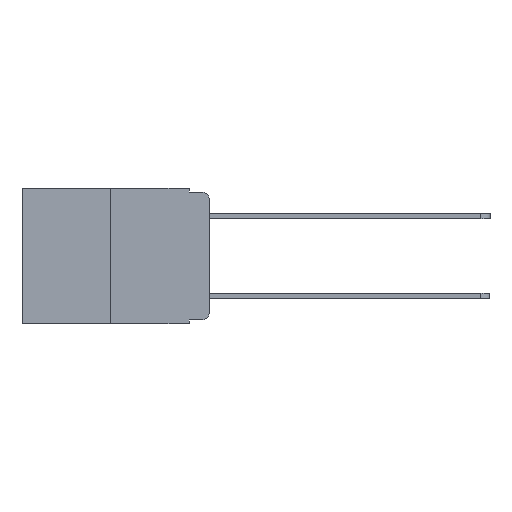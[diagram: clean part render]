
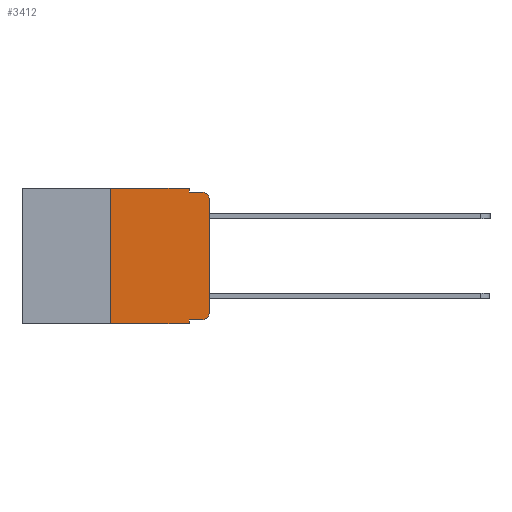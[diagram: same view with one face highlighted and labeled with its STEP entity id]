
A CAD part, left-side view. The second image highlights one B-rep face of the part: STEP entity #3412.
In plain terms, the highlighted planar face has unit normal (-1, 0, 0).
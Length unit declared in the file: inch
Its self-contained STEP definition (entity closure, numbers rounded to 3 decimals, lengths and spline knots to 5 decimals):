
#93 = LINE ( 'NONE', #2620, #12714 ) ;
#196 = CARTESIAN_POINT ( 'NONE',  ( 0., 0.051, -0.343 ) ) ;
#274 = VERTEX_POINT ( 'NONE', #10765 ) ;
#384 = LINE ( 'NONE', #11797, #10705 ) ;
#469 = CARTESIAN_POINT ( 'NONE',  ( 0., 0.051, -0.333 ) ) ;
#595 = VECTOR ( 'NONE', #872, 39.37008 ) ;
#602 = CARTESIAN_POINT ( 'NONE',  ( 0., 0.02, -0.03 ) ) ;
#603 = LINE ( 'NONE', #9924, #962 ) ;
#618 = EDGE_CURVE ( 'NONE', #274, #6680, #93, .T. ) ;
#852 = VERTEX_POINT ( 'NONE', #7088 ) ;
#872 = DIRECTION ( 'NONE',  ( 0., 0., -1. ) ) ;
#962 = VECTOR ( 'NONE', #9908, 39.37008 ) ;
#974 = CARTESIAN_POINT ( 'NONE',  ( 0., 0., -0.03 ) ) ;
#1253 = LINE ( 'NONE', #10570, #11458 ) ;
#1370 = EDGE_CURVE ( 'NONE', #6028, #9421, #603, .T. ) ;
#1397 = DIRECTION ( 'NONE',  ( 1., 0., 0. ) ) ;
#1731 = DIRECTION ( 'NONE',  ( 0., 0., -1. ) ) ;
#1858 = EDGE_CURVE ( 'NONE', #9421, #852, #7099, .T. ) ;
#1941 = DIRECTION ( 'NONE',  ( -1., 0., 0. ) ) ;
#2057 = ORIENTED_EDGE ( 'NONE', *, *, #3520, .T. ) ;
#2091 = VECTOR ( 'NONE', #4419, 39.37008 ) ;
#2113 = EDGE_CURVE ( 'NONE', #852, #6339, #10576, .T. ) ;
#2313 = ORIENTED_EDGE ( 'NONE', *, *, #1858, .F. ) ;
#2390 = ORIENTED_EDGE ( 'NONE', *, *, #618, .F. ) ;
#2583 = ORIENTED_EDGE ( 'NONE', *, *, #2706, .T. ) ;
#2620 = CARTESIAN_POINT ( 'NONE',  ( 0., 0.051, 0. ) ) ;
#2706 = EDGE_CURVE ( 'NONE', #6028, #6680, #384, .T. ) ;
#2750 = ORIENTED_EDGE ( 'NONE', *, *, #1370, .F. ) ;
#2766 = ORIENTED_EDGE ( 'NONE', *, *, #2113, .F. ) ;
#2822 = ORIENTED_EDGE ( 'NONE', *, *, #2831, .F. ) ;
#2831 = EDGE_CURVE ( 'NONE', #6339, #3176, #1253, .T. ) ;
#2878 = ORIENTED_EDGE ( 'NONE', *, *, #12180, .T. ) ;
#3176 = VERTEX_POINT ( 'NONE', #8554 ) ;
#3377 = CARTESIAN_POINT ( 'NONE',  ( 0., 0.02, -0.333 ) ) ;
#3412 = ADVANCED_FACE ( 'NONE', ( #4945 ), #4477, .F. ) ;
#3520 = EDGE_CURVE ( 'NONE', #12311, #3176, #8286, .T. ) ;
#3617 = ORIENTED_EDGE ( 'NONE', *, *, #12811, .T. ) ;
#3780 = AXIS2_PLACEMENT_3D ( 'NONE', #7839, #1941, #8841 ) ;
#4025 = VECTOR ( 'NONE', #11397, 39.37008 ) ;
#4159 = EDGE_CURVE ( 'NONE', #8027, #12311, #4782, .T. ) ;
#4335 = ORIENTED_EDGE ( 'NONE', *, *, #4159, .T. ) ;
#4419 = DIRECTION ( 'NONE',  ( 0., 0., 1. ) ) ;
#4477 = PLANE ( 'NONE',  #7040 ) ;
#4546 = VECTOR ( 'NONE', #9427, 39.37008 ) ;
#4782 = LINE ( 'NONE', #12189, #2091 ) ;
#4945 = FACE_OUTER_BOUND ( 'NONE', #6995, .T. ) ;
#6028 = VERTEX_POINT ( 'NONE', #11448 ) ;
#6165 = AXIS2_PLACEMENT_3D ( 'NONE', #602, #7662, #1731 ) ;
#6339 = VERTEX_POINT ( 'NONE', #10851 ) ;
#6680 = VERTEX_POINT ( 'NONE', #196 ) ;
#6995 = EDGE_LOOP ( 'NONE', ( #4335, #2057, #2822, #2766, #2313, #2750, #2583, #2390, #3617, #2878 ) ) ;
#7040 = AXIS2_PLACEMENT_3D ( 'NONE', #7373, #1397, #8377 ) ;
#7088 = CARTESIAN_POINT ( 'NONE',  ( 0., 0.051, 0. ) ) ;
#7099 = LINE ( 'NONE', #10105, #4546 ) ;
#7373 = CARTESIAN_POINT ( 'NONE',  ( 0., 0.473, 0. ) ) ;
#7648 = DIRECTION ( 'NONE',  ( 0., -1., 0. ) ) ;
#7662 = DIRECTION ( 'NONE',  ( -1., 0., 0. ) ) ;
#7782 = VERTEX_POINT ( 'NONE', #3377 ) ;
#7839 = CARTESIAN_POINT ( 'NONE',  ( 0., 0.02, -0.313 ) ) ;
#8027 = VERTEX_POINT ( 'NONE', #8509 ) ;
#8286 = CIRCLE ( 'NONE', #6165, 0.02 ) ;
#8377 = DIRECTION ( 'NONE',  ( 0., 0., -1. ) ) ;
#8509 = CARTESIAN_POINT ( 'NONE',  ( 0., 0., -0.313 ) ) ;
#8554 = CARTESIAN_POINT ( 'NONE',  ( 0., 0.02, -0.01 ) ) ;
#8841 = DIRECTION ( 'NONE',  ( 0., 0., -1. ) ) ;
#9421 = VERTEX_POINT ( 'NONE', #11928 ) ;
#9427 = DIRECTION ( 'NONE',  ( 0., -1., 0. ) ) ;
#9584 = DIRECTION ( 'NONE',  ( 0., 0., -1. ) ) ;
#9908 = DIRECTION ( 'NONE',  ( 0., 0., 1. ) ) ;
#9924 = CARTESIAN_POINT ( 'NONE',  ( 0., 0.25, 0. ) ) ;
#10075 = CIRCLE ( 'NONE', #3780, 0.02 ) ;
#10105 = CARTESIAN_POINT ( 'NONE',  ( 0., 0.473, 0. ) ) ;
#10570 = CARTESIAN_POINT ( 'NONE',  ( 0., 0.051, -0.01 ) ) ;
#10576 = LINE ( 'NONE', #12765, #595 ) ;
#10705 = VECTOR ( 'NONE', #11783, 39.37008 ) ;
#10765 = CARTESIAN_POINT ( 'NONE',  ( 0., 0.051, -0.333 ) ) ;
#10851 = CARTESIAN_POINT ( 'NONE',  ( 0., 0.051, -0.01 ) ) ;
#11397 = DIRECTION ( 'NONE',  ( 0., -1., 0. ) ) ;
#11448 = CARTESIAN_POINT ( 'NONE',  ( 0., 0.25, -0.343 ) ) ;
#11458 = VECTOR ( 'NONE', #7648, 39.37008 ) ;
#11737 = LINE ( 'NONE', #469, #4025 ) ;
#11783 = DIRECTION ( 'NONE',  ( 0., -1., 0. ) ) ;
#11797 = CARTESIAN_POINT ( 'NONE',  ( 0., 0.473, -0.343 ) ) ;
#11928 = CARTESIAN_POINT ( 'NONE',  ( 0., 0.25, 0. ) ) ;
#12180 = EDGE_CURVE ( 'NONE', #7782, #8027, #10075, .T. ) ;
#12189 = CARTESIAN_POINT ( 'NONE',  ( 0., 0., 0. ) ) ;
#12311 = VERTEX_POINT ( 'NONE', #974 ) ;
#12714 = VECTOR ( 'NONE', #9584, 39.37008 ) ;
#12765 = CARTESIAN_POINT ( 'NONE',  ( 0., 0.051, 0. ) ) ;
#12811 = EDGE_CURVE ( 'NONE', #274, #7782, #11737, .T. ) ;
